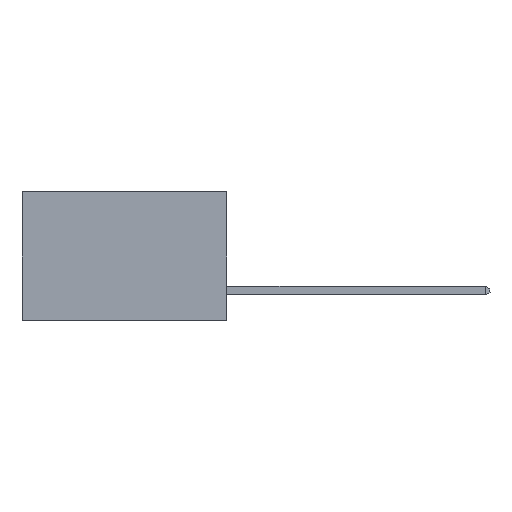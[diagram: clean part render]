
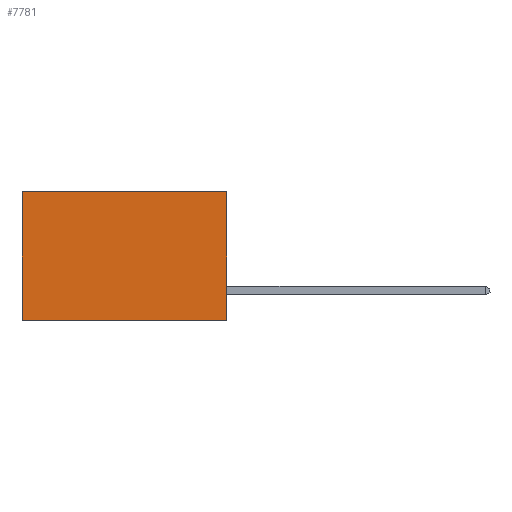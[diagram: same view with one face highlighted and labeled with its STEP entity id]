
A CAD part, left-side view. The second image highlights one B-rep face of the part: STEP entity #7781.
In plain terms, the highlighted planar face has unit normal (-1, 0, 0).
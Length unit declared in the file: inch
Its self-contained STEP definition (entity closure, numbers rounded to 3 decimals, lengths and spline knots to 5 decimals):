
#600 = ORIENTED_EDGE ( 'NONE', *, *, #1462, .T. ) ;
#618 = ORIENTED_EDGE ( 'NONE', *, *, #8311, .F. ) ;
#670 = ORIENTED_EDGE ( 'NONE', *, *, #6679, .F. ) ;
#737 = LINE ( 'NONE', #8064, #7186 ) ;
#774 = ORIENTED_EDGE ( 'NONE', *, *, #2196, .T. ) ;
#1462 = EDGE_CURVE ( 'NONE', #3070, #1936, #737, .T. ) ;
#1579 = FACE_OUTER_BOUND ( 'NONE', #5713, .T. ) ;
#1936 = VERTEX_POINT ( 'NONE', #5380 ) ;
#2196 = EDGE_CURVE ( 'NONE', #7882, #3070, #10773, .T. ) ;
#2552 = LINE ( 'NONE', #8655, #9019 ) ;
#3038 = CARTESIAN_POINT ( 'NONE',  ( 0.277, 0., 0. ) ) ;
#3070 = VERTEX_POINT ( 'NONE', #9279 ) ;
#3320 = AXIS2_PLACEMENT_3D ( 'NONE', #9464, #10269, #5404 ) ;
#4389 = LINE ( 'NONE', #6365, #10672 ) ;
#5380 = CARTESIAN_POINT ( 'NONE',  ( 0.277, 0.59, -0.37 ) ) ;
#5404 = DIRECTION ( 'NONE',  ( 0., 0., -1. ) ) ;
#5553 = VERTEX_POINT ( 'NONE', #7694 ) ;
#5713 = EDGE_LOOP ( 'NONE', ( #600, #618, #670, #774 ) ) ;
#5837 = DIRECTION ( 'NONE',  ( 0., 1., 0. ) ) ;
#6316 = DIRECTION ( 'NONE',  ( 0., 0., -1. ) ) ;
#6365 = CARTESIAN_POINT ( 'NONE',  ( 0.277, 0., -0.37 ) ) ;
#6679 = EDGE_CURVE ( 'NONE', #7882, #5553, #4389, .T. ) ;
#7186 = VECTOR ( 'NONE', #8040, 39.37008 ) ;
#7694 = CARTESIAN_POINT ( 'NONE',  ( 0.277, 0., -0.37 ) ) ;
#7781 = ADVANCED_FACE ( 'NONE', ( #1579 ), #8666, .F. ) ;
#7882 = VERTEX_POINT ( 'NONE', #10376 ) ;
#7912 = DIRECTION ( 'NONE',  ( 0., 1., 0. ) ) ;
#8040 = DIRECTION ( 'NONE',  ( 0., 0., -1. ) ) ;
#8064 = CARTESIAN_POINT ( 'NONE',  ( 0.277, 0.59, -0.37 ) ) ;
#8311 = EDGE_CURVE ( 'NONE', #5553, #1936, #2552, .T. ) ;
#8655 = CARTESIAN_POINT ( 'NONE',  ( 0.277, 0., -0.37 ) ) ;
#8666 = PLANE ( 'NONE',  #3320 ) ;
#9019 = VECTOR ( 'NONE', #7912, 39.37008 ) ;
#9279 = CARTESIAN_POINT ( 'NONE',  ( 0.277, 0.59, 0. ) ) ;
#9464 = CARTESIAN_POINT ( 'NONE',  ( 0.277, 0., -0.37 ) ) ;
#10269 = DIRECTION ( 'NONE',  ( 1., 0., 0. ) ) ;
#10376 = CARTESIAN_POINT ( 'NONE',  ( 0.277, 0., 0. ) ) ;
#10526 = VECTOR ( 'NONE', #5837, 39.37008 ) ;
#10672 = VECTOR ( 'NONE', #6316, 39.37008 ) ;
#10773 = LINE ( 'NONE', #3038, #10526 ) ;
